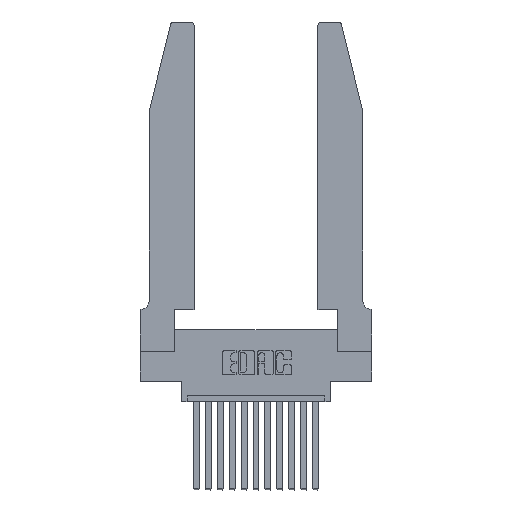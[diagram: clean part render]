
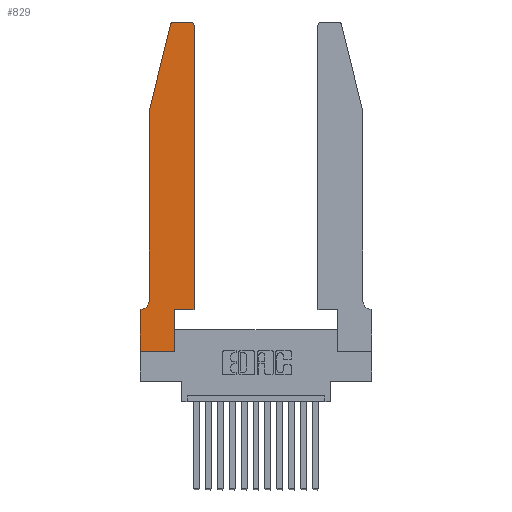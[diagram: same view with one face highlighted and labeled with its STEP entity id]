
A CAD part, top view. The second image highlights one B-rep face of the part: STEP entity #829.
In plain terms, the highlighted planar face has unit normal (0, 0, 1).
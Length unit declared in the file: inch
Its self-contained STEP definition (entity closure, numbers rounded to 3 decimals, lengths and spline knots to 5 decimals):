
#466 = DIRECTION ( 'NONE',  ( -0.239, -0.971, 0. ) ) ;
#479 = DIRECTION ( 'NONE',  ( 0., 1., 0. ) ) ;
#505 = LINE ( 'NONE', #2567, #2419 ) ;
#631 = CARTESIAN_POINT ( 'NONE',  ( 0., 0., 0.37 ) ) ;
#657 = DIRECTION ( 'NONE',  ( 0., 0., -1. ) ) ;
#680 = EDGE_LOOP ( 'NONE', ( #10607, #7433, #3881, #6747, #8304, #6653, #14750, #12771, #13015, #16438, #14115, #6845 ) ) ;
#719 = CARTESIAN_POINT ( 'NONE',  ( 0., 0.35, 0.37 ) ) ;
#721 = CARTESIAN_POINT ( 'NONE',  ( 0.0055, 0.42, 0.37 ) ) ;
#829 = ADVANCED_FACE ( 'NONE', ( #14657 ), #5437, .T. ) ;
#944 = DIRECTION ( 'NONE',  ( 1., 0., 0. ) ) ;
#1048 = CARTESIAN_POINT ( 'NONE',  ( 0.4505, 0.35, 0.37 ) ) ;
#1061 = CARTESIAN_POINT ( 'NONE',  ( 0.25487, 2.72718, 0.37 ) ) ;
#1069 = EDGE_CURVE ( 'NONE', #4835, #1501, #9230, .T. ) ;
#1162 = VECTOR ( 'NONE', #479, 39.37008 ) ;
#1188 = DIRECTION ( 'NONE',  ( 0., -1., 0. ) ) ;
#1220 = VERTEX_POINT ( 'NONE', #1048 ) ;
#1501 = VERTEX_POINT ( 'NONE', #15980 ) ;
#2228 = EDGE_CURVE ( 'NONE', #1220, #9245, #2866, .T. ) ;
#2353 = CARTESIAN_POINT ( 'NONE',  ( 0.2865, 0., 0.37 ) ) ;
#2419 = VECTOR ( 'NONE', #5376, 39.37008 ) ;
#2453 = AXIS2_PLACEMENT_3D ( 'NONE', #721, #657, #7129 ) ;
#2490 = DIRECTION ( 'NONE',  ( 0., 0., 1. ) ) ;
#2541 = AXIS2_PLACEMENT_3D ( 'NONE', #719, #11246, #8558 ) ;
#2567 = CARTESIAN_POINT ( 'NONE',  ( 0.2865, 0.35, 0.37 ) ) ;
#2629 = CARTESIAN_POINT ( 'NONE',  ( 0., 0., 0.37 ) ) ;
#2683 = VERTEX_POINT ( 'NONE', #2353 ) ;
#2866 = LINE ( 'NONE', #4445, #1162 ) ;
#3064 = VECTOR ( 'NONE', #944, 39.37008 ) ;
#3112 = VECTOR ( 'NONE', #5299, 39.37008 ) ;
#3566 = VECTOR ( 'NONE', #8115, 39.37008 ) ;
#3881 = ORIENTED_EDGE ( 'NONE', *, *, #10496, .T. ) ;
#4445 = CARTESIAN_POINT ( 'NONE',  ( 0.4505, 0.35, 0.37 ) ) ;
#4515 = CIRCLE ( 'NONE', #2453, 0.07 ) ;
#4687 = EDGE_CURVE ( 'NONE', #6691, #2683, #13177, .T. ) ;
#4835 = VERTEX_POINT ( 'NONE', #14768 ) ;
#4975 = CARTESIAN_POINT ( 'NONE',  ( 0.0755, 0.42, 0.37 ) ) ;
#5104 = VERTEX_POINT ( 'NONE', #8856 ) ;
#5116 = EDGE_CURVE ( 'NONE', #15364, #11205, #7583, .T. ) ;
#5153 = EDGE_CURVE ( 'NONE', #11205, #4835, #4515, .T. ) ;
#5299 = DIRECTION ( 'NONE',  ( 1., 0., 0. ) ) ;
#5376 = DIRECTION ( 'NONE',  ( 0., 1., 0. ) ) ;
#5437 = PLANE ( 'NONE',  #2541 ) ;
#5541 = CIRCLE ( 'NONE', #6835, 0.03 ) ;
#5651 = EDGE_CURVE ( 'NONE', #14629, #8695, #5541, .T. ) ;
#5959 = LINE ( 'NONE', #17160, #16083 ) ;
#6052 = CARTESIAN_POINT ( 'NONE',  ( 0.4505, 0.35, 0.37 ) ) ;
#6319 = EDGE_CURVE ( 'NONE', #5104, #1220, #8974, .T. ) ;
#6342 = AXIS2_PLACEMENT_3D ( 'NONE', #15581, #2490, #6493 ) ;
#6493 = DIRECTION ( 'NONE',  ( 1., 0., 0. ) ) ;
#6653 = ORIENTED_EDGE ( 'NONE', *, *, #1069, .T. ) ;
#6691 = VERTEX_POINT ( 'NONE', #2629 ) ;
#6747 = ORIENTED_EDGE ( 'NONE', *, *, #5116, .T. ) ;
#6835 = AXIS2_PLACEMENT_3D ( 'NONE', #14082, #16963, #14257 ) ;
#6845 = ORIENTED_EDGE ( 'NONE', *, *, #9843, .T. ) ;
#7091 = CARTESIAN_POINT ( 'NONE',  ( 0.0755, 2., 0.37 ) ) ;
#7129 = DIRECTION ( 'NONE',  ( -1., 0., 0. ) ) ;
#7433 = ORIENTED_EDGE ( 'NONE', *, *, #5651, .T. ) ;
#7583 = LINE ( 'NONE', #9069, #15675 ) ;
#7833 = CARTESIAN_POINT ( 'NONE',  ( 0.4205, 2.75, 0.37 ) ) ;
#7969 = VERTEX_POINT ( 'NONE', #7833 ) ;
#8115 = DIRECTION ( 'NONE',  ( -1., 0., 0. ) ) ;
#8304 = ORIENTED_EDGE ( 'NONE', *, *, #5153, .T. ) ;
#8558 = DIRECTION ( 'NONE',  ( 1., 0., 0. ) ) ;
#8695 = VERTEX_POINT ( 'NONE', #1061 ) ;
#8856 = CARTESIAN_POINT ( 'NONE',  ( 0.2865, 0.35, 0.37 ) ) ;
#8974 = LINE ( 'NONE', #6052, #3064 ) ;
#9069 = CARTESIAN_POINT ( 'NONE',  ( 0.0755, 2., 0.37 ) ) ;
#9217 = CARTESIAN_POINT ( 'NONE',  ( 0., 0., 0.37 ) ) ;
#9230 = LINE ( 'NONE', #10730, #15896 ) ;
#9245 = VERTEX_POINT ( 'NONE', #9711 ) ;
#9382 = EDGE_CURVE ( 'NONE', #7969, #14629, #9696, .T. ) ;
#9696 = LINE ( 'NONE', #15943, #3566 ) ;
#9711 = CARTESIAN_POINT ( 'NONE',  ( 0.4505, 2.72, 0.37 ) ) ;
#9843 = EDGE_CURVE ( 'NONE', #9245, #7969, #12781, .T. ) ;
#10496 = EDGE_CURVE ( 'NONE', #8695, #15364, #5959, .T. ) ;
#10607 = ORIENTED_EDGE ( 'NONE', *, *, #9382, .T. ) ;
#10614 = DIRECTION ( 'NONE',  ( -1., 0., 0. ) ) ;
#10730 = CARTESIAN_POINT ( 'NONE',  ( 0.0755, 0.35, 0.37 ) ) ;
#11205 = VERTEX_POINT ( 'NONE', #4975 ) ;
#11246 = DIRECTION ( 'NONE',  ( 0., 0., 1. ) ) ;
#12771 = ORIENTED_EDGE ( 'NONE', *, *, #4687, .T. ) ;
#12781 = CIRCLE ( 'NONE', #6342, 0.03 ) ;
#12944 = EDGE_CURVE ( 'NONE', #2683, #5104, #505, .T. ) ;
#13015 = ORIENTED_EDGE ( 'NONE', *, *, #12944, .T. ) ;
#13177 = LINE ( 'NONE', #9217, #3112 ) ;
#13467 = LINE ( 'NONE', #631, #14076 ) ;
#14076 = VECTOR ( 'NONE', #15216, 39.37008 ) ;
#14082 = CARTESIAN_POINT ( 'NONE',  ( 0.284, 2.72, 0.37 ) ) ;
#14115 = ORIENTED_EDGE ( 'NONE', *, *, #2228, .T. ) ;
#14257 = DIRECTION ( 'NONE',  ( 1., 0., 0. ) ) ;
#14629 = VERTEX_POINT ( 'NONE', #16027 ) ;
#14657 = FACE_OUTER_BOUND ( 'NONE', #680, .T. ) ;
#14750 = ORIENTED_EDGE ( 'NONE', *, *, #14882, .T. ) ;
#14768 = CARTESIAN_POINT ( 'NONE',  ( 0.0055, 0.35, 0.37 ) ) ;
#14882 = EDGE_CURVE ( 'NONE', #1501, #6691, #13467, .T. ) ;
#15216 = DIRECTION ( 'NONE',  ( 0., -1., 0. ) ) ;
#15364 = VERTEX_POINT ( 'NONE', #7091 ) ;
#15581 = CARTESIAN_POINT ( 'NONE',  ( 0.4205, 2.72, 0.37 ) ) ;
#15675 = VECTOR ( 'NONE', #1188, 39.37008 ) ;
#15896 = VECTOR ( 'NONE', #10614, 39.37008 ) ;
#15943 = CARTESIAN_POINT ( 'NONE',  ( 0.2605, 2.75, 0.37 ) ) ;
#15980 = CARTESIAN_POINT ( 'NONE',  ( 0., 0.35, 0.37 ) ) ;
#16027 = CARTESIAN_POINT ( 'NONE',  ( 0.284, 2.75, 0.37 ) ) ;
#16083 = VECTOR ( 'NONE', #466, 39.37008 ) ;
#16438 = ORIENTED_EDGE ( 'NONE', *, *, #6319, .T. ) ;
#16963 = DIRECTION ( 'NONE',  ( 0., 0., 1. ) ) ;
#17160 = CARTESIAN_POINT ( 'NONE',  ( 0.0755, 2., 0.37 ) ) ;
